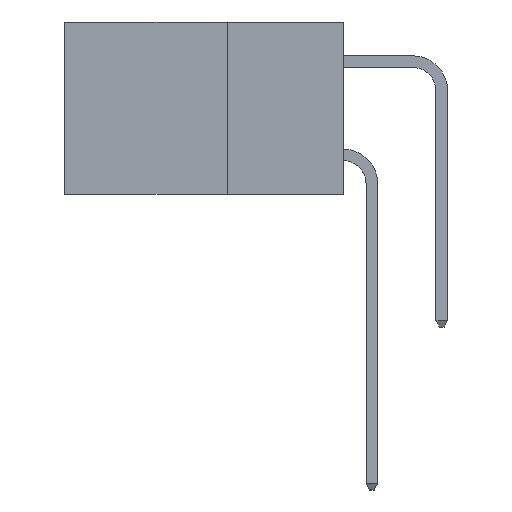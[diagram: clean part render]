
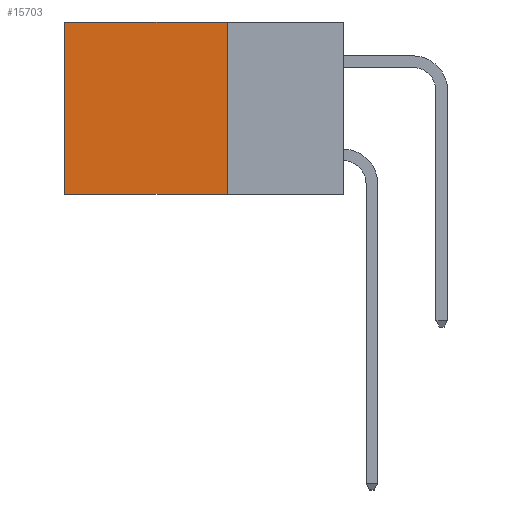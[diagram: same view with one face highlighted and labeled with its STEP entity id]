
A CAD part, left-side view. The second image highlights one B-rep face of the part: STEP entity #15703.
In plain terms, the highlighted planar face has unit normal (-1, 0, 0).
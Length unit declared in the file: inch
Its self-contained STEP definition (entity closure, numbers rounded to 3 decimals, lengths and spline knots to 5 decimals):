
#104 = EDGE_CURVE ( 'NONE', #14437, #15689, #13657, .T. ) ;
#921 = CARTESIAN_POINT ( 'NONE',  ( 0.2615, 0.6, -0.37 ) ) ;
#1642 = CARTESIAN_POINT ( 'NONE',  ( 0.2615, 0.25, 0. ) ) ;
#1754 = EDGE_CURVE ( 'NONE', #6987, #6278, #14186, .T. ) ;
#4150 = VECTOR ( 'NONE', #8127, 39.37008 ) ;
#4297 = EDGE_LOOP ( 'NONE', ( #5198, #9388, #14123, #11263 ) ) ;
#5198 = ORIENTED_EDGE ( 'NONE', *, *, #1754, .T. ) ;
#5592 = LINE ( 'NONE', #6422, #11828 ) ;
#5730 = DIRECTION ( 'NONE',  ( 0., 0., -1. ) ) ;
#6278 = VERTEX_POINT ( 'NONE', #921 ) ;
#6357 = DIRECTION ( 'NONE',  ( 0., 1., 0. ) ) ;
#6422 = CARTESIAN_POINT ( 'NONE',  ( 0.2615, 0.25, 0. ) ) ;
#6987 = VERTEX_POINT ( 'NONE', #11378 ) ;
#7106 = CARTESIAN_POINT ( 'NONE',  ( 0.2615, 0.25, -0.37 ) ) ;
#7140 = DIRECTION ( 'NONE',  ( 0., 1., 0. ) ) ;
#7155 = VECTOR ( 'NONE', #7140, 39.37008 ) ;
#8127 = DIRECTION ( 'NONE',  ( 0., 0., -1. ) ) ;
#9388 = ORIENTED_EDGE ( 'NONE', *, *, #12148, .F. ) ;
#9511 = CARTESIAN_POINT ( 'NONE',  ( 0.2615, 0.25, -0.37 ) ) ;
#9579 = FACE_OUTER_BOUND ( 'NONE', #4297, .T. ) ;
#9713 = DIRECTION ( 'NONE',  ( 0., 0., -1. ) ) ;
#9716 = DIRECTION ( 'NONE',  ( 1., 0., 0. ) ) ;
#9761 = CARTESIAN_POINT ( 'NONE',  ( 0.2615, 0.25, -0.37 ) ) ;
#9807 = PLANE ( 'NONE',  #15403 ) ;
#10156 = CARTESIAN_POINT ( 'NONE',  ( 0.2615, 0.25, -0.37 ) ) ;
#10942 = VECTOR ( 'NONE', #5730, 39.37008 ) ;
#11263 = ORIENTED_EDGE ( 'NONE', *, *, #15950, .T. ) ;
#11378 = CARTESIAN_POINT ( 'NONE',  ( 0.2615, 0.6, 0. ) ) ;
#11828 = VECTOR ( 'NONE', #6357, 39.37008 ) ;
#12148 = EDGE_CURVE ( 'NONE', #15689, #6278, #13654, .T. ) ;
#13654 = LINE ( 'NONE', #7106, #7155 ) ;
#13657 = LINE ( 'NONE', #9511, #4150 ) ;
#14123 = ORIENTED_EDGE ( 'NONE', *, *, #104, .F. ) ;
#14186 = LINE ( 'NONE', #15074, #10942 ) ;
#14437 = VERTEX_POINT ( 'NONE', #1642 ) ;
#15074 = CARTESIAN_POINT ( 'NONE',  ( 0.2615, 0.6, -0.37 ) ) ;
#15403 = AXIS2_PLACEMENT_3D ( 'NONE', #9761, #9716, #9713 ) ;
#15689 = VERTEX_POINT ( 'NONE', #10156 ) ;
#15703 = ADVANCED_FACE ( 'NONE', ( #9579 ), #9807, .F. ) ;
#15950 = EDGE_CURVE ( 'NONE', #14437, #6987, #5592, .T. ) ;
